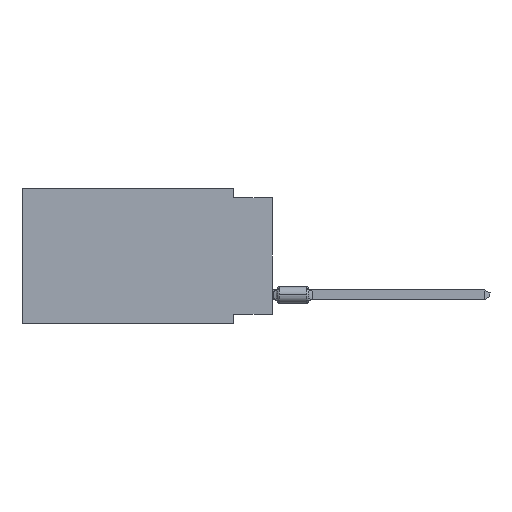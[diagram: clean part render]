
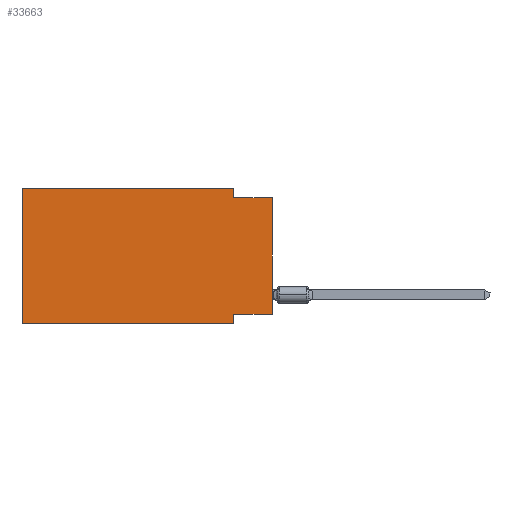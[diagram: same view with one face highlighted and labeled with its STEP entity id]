
A CAD part, left-side view. The second image highlights one B-rep face of the part: STEP entity #33663.
In plain terms, the highlighted planar face has unit normal (-1, 0, 0).
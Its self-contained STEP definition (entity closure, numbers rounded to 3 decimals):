
#6687 = CARTESIAN_POINT ( 'NONE',  ( 0., 0., 0. ) ) ;
#10747 = CARTESIAN_POINT ( 'NONE',  ( 0., 0., -0.635 ) ) ;
#12499 = CARTESIAN_POINT ( 'NONE',  ( 0., 16.383, -8.89 ) ) ;
#13524 = LINE ( 'NONE', #66305, #42909 ) ;
#14380 = EDGE_CURVE ( 'NONE', #48783, #74038, #44428, .T. ) ;
#14400 = AXIS2_PLACEMENT_3D ( 'NONE', #59998, #91206, #21097 ) ;
#15853 = VERTEX_POINT ( 'NONE', #51440 ) ;
#21097 = DIRECTION ( 'NONE',  ( 0., 0., -1. ) ) ;
#24473 = VECTOR ( 'NONE', #28027, 1000. ) ;
#27413 = VECTOR ( 'NONE', #65004, 1000. ) ;
#28027 = DIRECTION ( 'NONE',  ( 0., 0., -1. ) ) ;
#28780 = PLANE ( 'NONE',  #14400 ) ;
#30045 = EDGE_CURVE ( 'NONE', #48218, #68479, #37565, .T. ) ;
#33034 = LINE ( 'NONE', #64252, #39293 ) ;
#33270 = DIRECTION ( 'NONE',  ( 0., -1., 0. ) ) ;
#33663 = ADVANCED_FACE ( 'NONE', ( #98861 ), #28780, .F. ) ;
#36737 = DIRECTION ( 'NONE',  ( 0., 0., 1. ) ) ;
#37464 = ORIENTED_EDGE ( 'NONE', *, *, #72273, .T. ) ;
#37565 = LINE ( 'NONE', #71199, #93909 ) ;
#37687 = CARTESIAN_POINT ( 'NONE',  ( 0., 2.54, -8.89 ) ) ;
#38243 = EDGE_CURVE ( 'NONE', #74038, #15853, #13524, .T. ) ;
#39293 = VECTOR ( 'NONE', #57577, 1000. ) ;
#41783 = ORIENTED_EDGE ( 'NONE', *, *, #14380, .F. ) ;
#42909 = VECTOR ( 'NONE', #58606, 1000. ) ;
#44085 = VECTOR ( 'NONE', #36737, 1000. ) ;
#44428 = LINE ( 'NONE', #100149, #44085 ) ;
#45574 = LINE ( 'NONE', #6687, #70989 ) ;
#46262 = VERTEX_POINT ( 'NONE', #100804 ) ;
#46358 = VERTEX_POINT ( 'NONE', #87524 ) ;
#48218 = VERTEX_POINT ( 'NONE', #81239 ) ;
#48670 = DIRECTION ( 'NONE',  ( 0., 1., 0. ) ) ;
#48783 = VERTEX_POINT ( 'NONE', #12499 ) ;
#51050 = ORIENTED_EDGE ( 'NONE', *, *, #38243, .F. ) ;
#51440 = CARTESIAN_POINT ( 'NONE',  ( 0., 2.54, 0. ) ) ;
#51446 = EDGE_CURVE ( 'NONE', #48783, #92227, #72668, .T. ) ;
#54504 = EDGE_LOOP ( 'NONE', ( #37464, #84853, #96812, #51050, #41783, #55546, #80817, #79813 ) ) ;
#55546 = ORIENTED_EDGE ( 'NONE', *, *, #51446, .T. ) ;
#57272 = CARTESIAN_POINT ( 'NONE',  ( 0., 2.54, -8.89 ) ) ;
#57354 = EDGE_CURVE ( 'NONE', #46262, #46358, #64499, .T. ) ;
#57577 = DIRECTION ( 'NONE',  ( 0., 0., -1. ) ) ;
#58606 = DIRECTION ( 'NONE',  ( 0., -1., 0. ) ) ;
#59998 = CARTESIAN_POINT ( 'NONE',  ( 0., 16.383, 0. ) ) ;
#64252 = CARTESIAN_POINT ( 'NONE',  ( 0., 2.54, 0. ) ) ;
#64499 = LINE ( 'NONE', #10747, #27413 ) ;
#65004 = DIRECTION ( 'NONE',  ( 0., -1., 0. ) ) ;
#66305 = CARTESIAN_POINT ( 'NONE',  ( 0., 16.383, 0. ) ) ;
#67884 = CARTESIAN_POINT ( 'NONE',  ( 0., 2.54, -8.255 ) ) ;
#68479 = VERTEX_POINT ( 'NONE', #67884 ) ;
#69117 = DIRECTION ( 'NONE',  ( 0., 0., 1. ) ) ;
#70989 = VECTOR ( 'NONE', #69117, 1000. ) ;
#71199 = CARTESIAN_POINT ( 'NONE',  ( 0., 0., -8.255 ) ) ;
#72273 = EDGE_CURVE ( 'NONE', #48218, #46358, #45574, .T. ) ;
#72668 = LINE ( 'NONE', #94156, #88809 ) ;
#74038 = VERTEX_POINT ( 'NONE', #93766 ) ;
#74603 = LINE ( 'NONE', #37687, #24473 ) ;
#79813 = ORIENTED_EDGE ( 'NONE', *, *, #30045, .F. ) ;
#80817 = ORIENTED_EDGE ( 'NONE', *, *, #86377, .F. ) ;
#81239 = CARTESIAN_POINT ( 'NONE',  ( 0., 0., -8.255 ) ) ;
#84853 = ORIENTED_EDGE ( 'NONE', *, *, #57354, .F. ) ;
#85538 = EDGE_CURVE ( 'NONE', #15853, #46262, #33034, .T. ) ;
#86377 = EDGE_CURVE ( 'NONE', #68479, #92227, #74603, .T. ) ;
#87524 = CARTESIAN_POINT ( 'NONE',  ( 0., 0., -0.635 ) ) ;
#88809 = VECTOR ( 'NONE', #33270, 1000. ) ;
#91206 = DIRECTION ( 'NONE',  ( 1., 0., 0. ) ) ;
#92227 = VERTEX_POINT ( 'NONE', #57272 ) ;
#93766 = CARTESIAN_POINT ( 'NONE',  ( 0., 16.383, 0. ) ) ;
#93909 = VECTOR ( 'NONE', #48670, 1000. ) ;
#94156 = CARTESIAN_POINT ( 'NONE',  ( 0., 16.383, -8.89 ) ) ;
#96812 = ORIENTED_EDGE ( 'NONE', *, *, #85538, .F. ) ;
#98861 = FACE_OUTER_BOUND ( 'NONE', #54504, .T. ) ;
#100149 = CARTESIAN_POINT ( 'NONE',  ( 0., 16.383, 0. ) ) ;
#100804 = CARTESIAN_POINT ( 'NONE',  ( 0., 2.54, -0.635 ) ) ;
